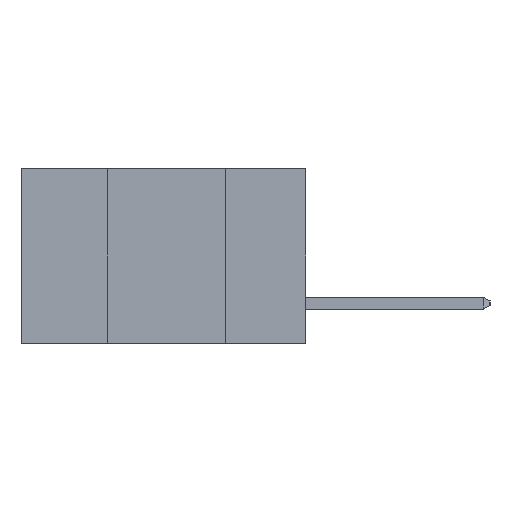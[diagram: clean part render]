
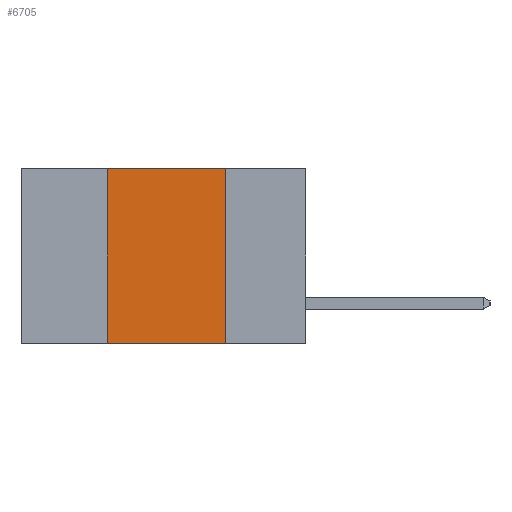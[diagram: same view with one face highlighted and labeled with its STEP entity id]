
A CAD part, left-side view. The second image highlights one B-rep face of the part: STEP entity #6705.
In plain terms, the highlighted planar face has unit normal (-1, 0, 0).
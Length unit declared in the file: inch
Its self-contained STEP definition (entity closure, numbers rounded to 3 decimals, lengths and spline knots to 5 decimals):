
#199 = EDGE_LOOP ( 'NONE', ( #8471, #1987, #9034, #4255 ) ) ;
#296 = EDGE_CURVE ( 'NONE', #4021, #11840, #8672, .T. ) ;
#640 = VECTOR ( 'NONE', #7935, 39.37008 ) ;
#792 = EDGE_CURVE ( 'NONE', #1965, #2649, #9214, .T. ) ;
#1216 = VECTOR ( 'NONE', #7404, 39.37008 ) ;
#1277 = LINE ( 'NONE', #7815, #8425 ) ;
#1965 = VERTEX_POINT ( 'NONE', #4758 ) ;
#1987 = ORIENTED_EDGE ( 'NONE', *, *, #296, .F. ) ;
#1993 = DIRECTION ( 'NONE',  ( 0., 0., -1. ) ) ;
#2649 = VERTEX_POINT ( 'NONE', #11588 ) ;
#3104 = DIRECTION ( 'NONE',  ( 0., -1., 0. ) ) ;
#3873 = AXIS2_PLACEMENT_3D ( 'NONE', #5114, #6046, #6090 ) ;
#4021 = VERTEX_POINT ( 'NONE', #4692 ) ;
#4255 = ORIENTED_EDGE ( 'NONE', *, *, #792, .T. ) ;
#4692 = CARTESIAN_POINT ( 'NONE',  ( 0., 0.42, 0. ) ) ;
#4758 = CARTESIAN_POINT ( 'NONE',  ( 0., 0.42, -0.37 ) ) ;
#5114 = CARTESIAN_POINT ( 'NONE',  ( 0., 0.6, 0. ) ) ;
#5847 = VECTOR ( 'NONE', #3104, 39.37008 ) ;
#6046 = DIRECTION ( 'NONE',  ( 1., 0., 0. ) ) ;
#6090 = DIRECTION ( 'NONE',  ( 0., 0., -1. ) ) ;
#6565 = EDGE_CURVE ( 'NONE', #11840, #2649, #1277, .T. ) ;
#6705 = ADVANCED_FACE ( 'NONE', ( #11484 ), #10678, .F. ) ;
#6998 = CARTESIAN_POINT ( 'NONE',  ( 0., 0.42, 0. ) ) ;
#7404 = DIRECTION ( 'NONE',  ( 0., -1., 0. ) ) ;
#7815 = CARTESIAN_POINT ( 'NONE',  ( 0., 0.17, 0. ) ) ;
#7935 = DIRECTION ( 'NONE',  ( 0., 0., 1. ) ) ;
#8137 = LINE ( 'NONE', #6998, #640 ) ;
#8425 = VECTOR ( 'NONE', #1993, 39.37008 ) ;
#8471 = ORIENTED_EDGE ( 'NONE', *, *, #6565, .F. ) ;
#8672 = LINE ( 'NONE', #9703, #1216 ) ;
#9034 = ORIENTED_EDGE ( 'NONE', *, *, #11594, .F. ) ;
#9214 = LINE ( 'NONE', #12050, #5847 ) ;
#9703 = CARTESIAN_POINT ( 'NONE',  ( 0., 0.6, 0. ) ) ;
#10198 = CARTESIAN_POINT ( 'NONE',  ( 0., 0.17, 0. ) ) ;
#10678 = PLANE ( 'NONE',  #3873 ) ;
#11484 = FACE_OUTER_BOUND ( 'NONE', #199, .T. ) ;
#11588 = CARTESIAN_POINT ( 'NONE',  ( 0., 0.17, -0.37 ) ) ;
#11594 = EDGE_CURVE ( 'NONE', #1965, #4021, #8137, .T. ) ;
#11840 = VERTEX_POINT ( 'NONE', #10198 ) ;
#12050 = CARTESIAN_POINT ( 'NONE',  ( 0., 0.6, -0.37 ) ) ;
